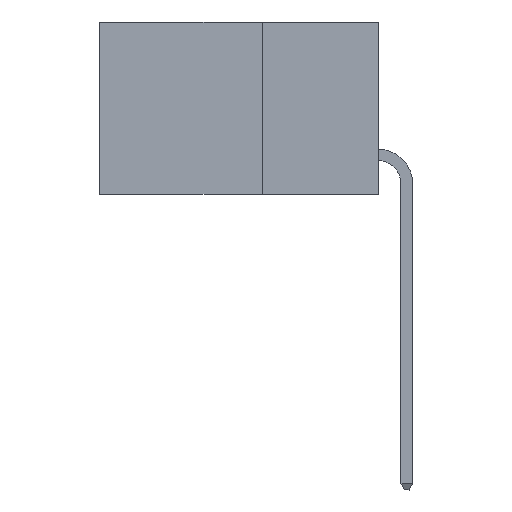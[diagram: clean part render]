
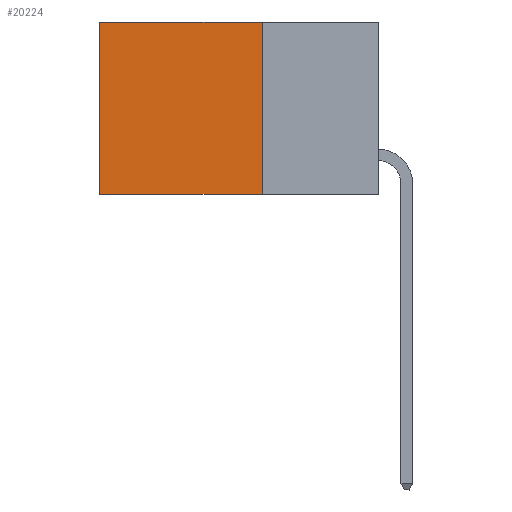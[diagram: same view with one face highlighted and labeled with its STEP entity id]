
A CAD part, left-side view. The second image highlights one B-rep face of the part: STEP entity #20224.
In plain terms, the highlighted planar face has unit normal (-1, 0, 0).
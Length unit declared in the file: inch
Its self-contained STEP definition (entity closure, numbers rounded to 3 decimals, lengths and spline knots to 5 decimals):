
#1428 = VERTEX_POINT ( 'NONE', #10139 ) ;
#1454 = CARTESIAN_POINT ( 'NONE',  ( 0.298, 0.25, -0.37 ) ) ;
#2523 = LINE ( 'NONE', #19341, #11704 ) ;
#2927 = AXIS2_PLACEMENT_3D ( 'NONE', #4367, #16897, #6213 ) ;
#3860 = ORIENTED_EDGE ( 'NONE', *, *, #8584, .F. ) ;
#3998 = DIRECTION ( 'NONE',  ( 0., 0., -1. ) ) ;
#4367 = CARTESIAN_POINT ( 'NONE',  ( 0.298, 0.25, 0. ) ) ;
#5852 = CARTESIAN_POINT ( 'NONE',  ( 0.298, 0.25, 0. ) ) ;
#6107 = LINE ( 'NONE', #1454, #14594 ) ;
#6213 = DIRECTION ( 'NONE',  ( 0., 0., -1. ) ) ;
#6640 = CARTESIAN_POINT ( 'NONE',  ( 0.298, 0.6, -0.37 ) ) ;
#6900 = DIRECTION ( 'NONE',  ( 0., 1., 0. ) ) ;
#6916 = VERTEX_POINT ( 'NONE', #13365 ) ;
#8170 = ORIENTED_EDGE ( 'NONE', *, *, #21396, .F. ) ;
#8584 = EDGE_CURVE ( 'NONE', #14506, #16558, #6107, .T. ) ;
#8588 = ORIENTED_EDGE ( 'NONE', *, *, #11040, .T. ) ;
#8745 = ORIENTED_EDGE ( 'NONE', *, *, #10711, .T. ) ;
#9609 = LINE ( 'NONE', #5852, #13870 ) ;
#9666 = DIRECTION ( 'NONE',  ( 0., 0., -1. ) ) ;
#9986 = VECTOR ( 'NONE', #9666, 39.37008 ) ;
#10139 = CARTESIAN_POINT ( 'NONE',  ( 0.298, 0.25, 0. ) ) ;
#10711 = EDGE_CURVE ( 'NONE', #6916, #16558, #19427, .T. ) ;
#11040 = EDGE_CURVE ( 'NONE', #1428, #6916, #2523, .T. ) ;
#11704 = VECTOR ( 'NONE', #6900, 39.37008 ) ;
#12400 = DIRECTION ( 'NONE',  ( 0., 1., 0. ) ) ;
#13365 = CARTESIAN_POINT ( 'NONE',  ( 0.298, 0.6, 0. ) ) ;
#13870 = VECTOR ( 'NONE', #3998, 39.37008 ) ;
#14506 = VERTEX_POINT ( 'NONE', #16554 ) ;
#14594 = VECTOR ( 'NONE', #12400, 39.37008 ) ;
#15178 = PLANE ( 'NONE',  #2927 ) ;
#16554 = CARTESIAN_POINT ( 'NONE',  ( 0.298, 0.25, -0.37 ) ) ;
#16558 = VERTEX_POINT ( 'NONE', #6640 ) ;
#16897 = DIRECTION ( 'NONE',  ( 1., 0., 0. ) ) ;
#19341 = CARTESIAN_POINT ( 'NONE',  ( 0.298, 0.25, 0. ) ) ;
#19427 = LINE ( 'NONE', #20264, #9986 ) ;
#20224 = ADVANCED_FACE ( 'NONE', ( #21578 ), #15178, .F. ) ;
#20264 = CARTESIAN_POINT ( 'NONE',  ( 0.298, 0.6, 0. ) ) ;
#21396 = EDGE_CURVE ( 'NONE', #1428, #14506, #9609, .T. ) ;
#21578 = FACE_OUTER_BOUND ( 'NONE', #22628, .T. ) ;
#22628 = EDGE_LOOP ( 'NONE', ( #8745, #3860, #8170, #8588 ) ) ;
